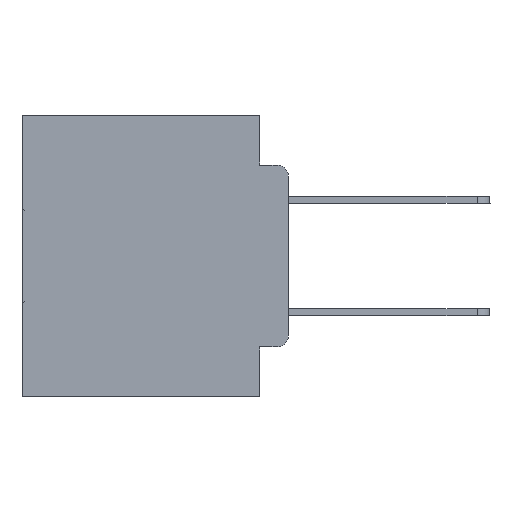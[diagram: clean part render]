
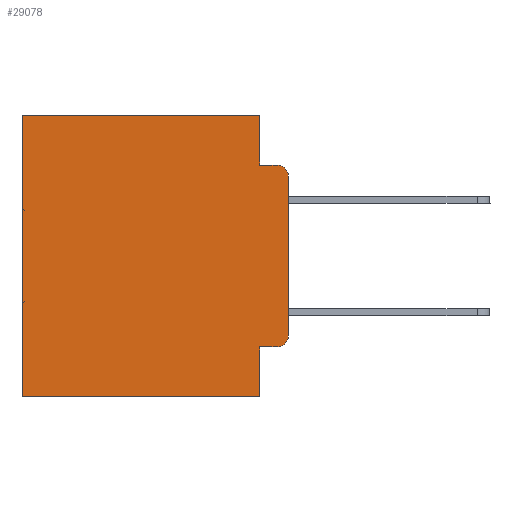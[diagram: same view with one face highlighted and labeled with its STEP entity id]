
A CAD part, left-side view. The second image highlights one B-rep face of the part: STEP entity #29078.
In plain terms, the highlighted planar face has unit normal (-1, 0, 0).
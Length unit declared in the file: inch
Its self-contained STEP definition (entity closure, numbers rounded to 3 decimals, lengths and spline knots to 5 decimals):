
#962 = DIRECTION ( 'NONE',  ( 0., 0., -1. ) ) ;
#998 = DIRECTION ( 'NONE',  ( -1., 0., 0. ) ) ;
#1774 = ORIENTED_EDGE ( 'NONE', *, *, #10005, .T. ) ;
#1836 = VECTOR ( 'NONE', #21622, 39.37008 ) ;
#1971 = ORIENTED_EDGE ( 'NONE', *, *, #7012, .T. ) ;
#2139 = EDGE_CURVE ( 'NONE', #6847, #15991, #8936, .T. ) ;
#3389 = VERTEX_POINT ( 'NONE', #7224 ) ;
#3906 = LINE ( 'NONE', #14986, #30532 ) ;
#3968 = CARTESIAN_POINT ( 'NONE',  ( 0.298, 0.051, -0.0885 ) ) ;
#4083 = CARTESIAN_POINT ( 'NONE',  ( 0.298, 0., 0. ) ) ;
#4140 = DIRECTION ( 'NONE',  ( -1., 0., 0. ) ) ;
#4249 = VERTEX_POINT ( 'NONE', #24810 ) ;
#4820 = CARTESIAN_POINT ( 'NONE',  ( 0.298, 0., 0. ) ) ;
#5082 = CARTESIAN_POINT ( 'NONE',  ( 0.298, 0., 0. ) ) ;
#5139 = CARTESIAN_POINT ( 'NONE',  ( 0.298, 0.02, -0.0885 ) ) ;
#5880 = LINE ( 'NONE', #28605, #25488 ) ;
#6169 = LINE ( 'NONE', #19213, #21060 ) ;
#6847 = VERTEX_POINT ( 'NONE', #15757 ) ;
#6855 = EDGE_CURVE ( 'NONE', #27843, #17181, #10999, .T. ) ;
#6932 = EDGE_CURVE ( 'NONE', #25781, #17181, #30936, .T. ) ;
#7012 = EDGE_CURVE ( 'NONE', #23673, #4249, #5880, .T. ) ;
#7224 = CARTESIAN_POINT ( 'NONE',  ( 0.298, 0.051, -0.4115 ) ) ;
#7439 = VERTEX_POINT ( 'NONE', #23264 ) ;
#8131 = LINE ( 'NONE', #4083, #1836 ) ;
#8315 = LINE ( 'NONE', #18178, #19259 ) ;
#8936 = CIRCLE ( 'NONE', #13128, 0.02 ) ;
#9027 = DIRECTION ( 'NONE',  ( 0., 0., -1. ) ) ;
#9214 = DIRECTION ( 'NONE',  ( 0., 0., -1. ) ) ;
#9314 = ORIENTED_EDGE ( 'NONE', *, *, #21860, .F. ) ;
#10005 = EDGE_CURVE ( 'NONE', #7439, #23673, #30288, .T. ) ;
#10299 = EDGE_CURVE ( 'NONE', #3389, #32099, #20477, .T. ) ;
#10999 = CIRCLE ( 'NONE', #17171, 0.02 ) ;
#11280 = CARTESIAN_POINT ( 'NONE',  ( 0.298, 0.473, 0. ) ) ;
#11883 = VECTOR ( 'NONE', #962, 39.37008 ) ;
#13128 = AXIS2_PLACEMENT_3D ( 'NONE', #16679, #4140, #9214 ) ;
#13180 = CARTESIAN_POINT ( 'NONE',  ( 0.298, 0.051, 0. ) ) ;
#13369 = VECTOR ( 'NONE', #14088, 39.37008 ) ;
#13599 = EDGE_LOOP ( 'NONE', ( #14817, #16952, #21293, #18845, #1774, #1971, #9314, #22488, #17889, #16751 ) ) ;
#14088 = DIRECTION ( 'NONE',  ( 0., -1., 0. ) ) ;
#14817 = ORIENTED_EDGE ( 'NONE', *, *, #28817, .F. ) ;
#14986 = CARTESIAN_POINT ( 'NONE',  ( 0.298, 0.051, 0. ) ) ;
#15757 = CARTESIAN_POINT ( 'NONE',  ( 0.298, 0.02, -0.4115 ) ) ;
#15762 = CARTESIAN_POINT ( 'NONE',  ( 0.298, 0., -0.3915 ) ) ;
#15839 = VECTOR ( 'NONE', #24805, 39.37008 ) ;
#15991 = VERTEX_POINT ( 'NONE', #15762 ) ;
#16679 = CARTESIAN_POINT ( 'NONE',  ( 0.298, 0.02, -0.3915 ) ) ;
#16751 = ORIENTED_EDGE ( 'NONE', *, *, #2139, .T. ) ;
#16952 = ORIENTED_EDGE ( 'NONE', *, *, #6855, .T. ) ;
#17171 = AXIS2_PLACEMENT_3D ( 'NONE', #23479, #998, #18537 ) ;
#17181 = VERTEX_POINT ( 'NONE', #5139 ) ;
#17889 = ORIENTED_EDGE ( 'NONE', *, *, #24775, .T. ) ;
#18178 = CARTESIAN_POINT ( 'NONE',  ( 0.298, 0.051, -0.4115 ) ) ;
#18537 = DIRECTION ( 'NONE',  ( 0., 0., -1. ) ) ;
#18845 = ORIENTED_EDGE ( 'NONE', *, *, #27005, .F. ) ;
#19213 = CARTESIAN_POINT ( 'NONE',  ( 0.298, 0., -0.5 ) ) ;
#19259 = VECTOR ( 'NONE', #24620, 39.37008 ) ;
#20180 = CARTESIAN_POINT ( 'NONE',  ( 0.298, 0.051, -0.5 ) ) ;
#20473 = CARTESIAN_POINT ( 'NONE',  ( 0.298, 0., -0.1085 ) ) ;
#20477 = LINE ( 'NONE', #13180, #11883 ) ;
#20609 = AXIS2_PLACEMENT_3D ( 'NONE', #4820, #22371, #27353 ) ;
#21060 = VECTOR ( 'NONE', #31580, 39.37008 ) ;
#21293 = ORIENTED_EDGE ( 'NONE', *, *, #6932, .F. ) ;
#21622 = DIRECTION ( 'NONE',  ( 0., 0., -1. ) ) ;
#21860 = EDGE_CURVE ( 'NONE', #32099, #4249, #6169, .T. ) ;
#22371 = DIRECTION ( 'NONE',  ( 1., 0., 0. ) ) ;
#22488 = ORIENTED_EDGE ( 'NONE', *, *, #10299, .F. ) ;
#23264 = CARTESIAN_POINT ( 'NONE',  ( 0.298, 0.051, 0. ) ) ;
#23479 = CARTESIAN_POINT ( 'NONE',  ( 0.298, 0.02, -0.1085 ) ) ;
#23673 = VERTEX_POINT ( 'NONE', #11280 ) ;
#24620 = DIRECTION ( 'NONE',  ( 0., -1., 0. ) ) ;
#24775 = EDGE_CURVE ( 'NONE', #3389, #6847, #8315, .T. ) ;
#24805 = DIRECTION ( 'NONE',  ( 0., 1., 0. ) ) ;
#24810 = CARTESIAN_POINT ( 'NONE',  ( 0.298, 0.473, -0.5 ) ) ;
#25488 = VECTOR ( 'NONE', #9027, 39.37008 ) ;
#25781 = VERTEX_POINT ( 'NONE', #29782 ) ;
#27005 = EDGE_CURVE ( 'NONE', #7439, #25781, #3906, .T. ) ;
#27353 = DIRECTION ( 'NONE',  ( 0., 0., -1. ) ) ;
#27843 = VERTEX_POINT ( 'NONE', #20473 ) ;
#28605 = CARTESIAN_POINT ( 'NONE',  ( 0.298, 0.473, 0. ) ) ;
#28817 = EDGE_CURVE ( 'NONE', #27843, #15991, #8131, .T. ) ;
#29078 = ADVANCED_FACE ( 'NONE', ( #30419 ), #32459, .F. ) ;
#29782 = CARTESIAN_POINT ( 'NONE',  ( 0.298, 0.051, -0.0885 ) ) ;
#30288 = LINE ( 'NONE', #5082, #15839 ) ;
#30419 = FACE_OUTER_BOUND ( 'NONE', #13599, .T. ) ;
#30532 = VECTOR ( 'NONE', #32343, 39.37008 ) ;
#30936 = LINE ( 'NONE', #3968, #13369 ) ;
#31580 = DIRECTION ( 'NONE',  ( 0., 1., 0. ) ) ;
#32099 = VERTEX_POINT ( 'NONE', #20180 ) ;
#32343 = DIRECTION ( 'NONE',  ( 0., 0., -1. ) ) ;
#32459 = PLANE ( 'NONE',  #20609 ) ;
